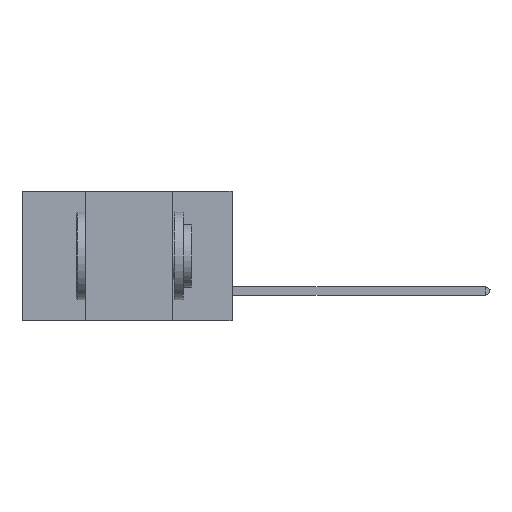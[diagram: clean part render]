
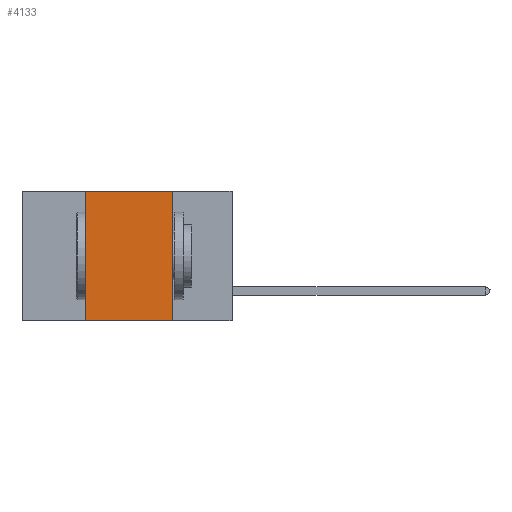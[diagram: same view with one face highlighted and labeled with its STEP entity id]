
A CAD part, left-side view. The second image highlights one B-rep face of the part: STEP entity #4133.
In plain terms, the highlighted planar face has unit normal (-1, 0, 0).
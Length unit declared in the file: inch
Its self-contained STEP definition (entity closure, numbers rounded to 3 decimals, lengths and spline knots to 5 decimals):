
#1001 = CARTESIAN_POINT ( 'NONE',  ( 0., 0.17, 0. ) ) ;
#1091 = ORIENTED_EDGE ( 'NONE', *, *, #10541, .T. ) ;
#1177 = EDGE_CURVE ( 'NONE', #11917, #10775, #2527, .T. ) ;
#1195 = CARTESIAN_POINT ( 'NONE',  ( 0., 0.6, 0. ) ) ;
#1341 = CARTESIAN_POINT ( 'NONE',  ( 0., 0.42, 0. ) ) ;
#2527 = LINE ( 'NONE', #1001, #4991 ) ;
#3161 = DIRECTION ( 'NONE',  ( 1., 0., 0. ) ) ;
#3175 = EDGE_LOOP ( 'NONE', ( #11600, #6607, #9332, #1091 ) ) ;
#3208 = VECTOR ( 'NONE', #3527, 39.37008 ) ;
#3527 = DIRECTION ( 'NONE',  ( 0., -1., 0. ) ) ;
#3568 = DIRECTION ( 'NONE',  ( 0., -1., 0. ) ) ;
#3571 = DIRECTION ( 'NONE',  ( 0., 0., 1. ) ) ;
#3637 = CARTESIAN_POINT ( 'NONE',  ( 0., 0.6, -0.37 ) ) ;
#3940 = DIRECTION ( 'NONE',  ( 0., 0., -1. ) ) ;
#4133 = ADVANCED_FACE ( 'NONE', ( #4643 ), #5069, .F. ) ;
#4355 = AXIS2_PLACEMENT_3D ( 'NONE', #1195, #3161, #6945 ) ;
#4589 = EDGE_CURVE ( 'NONE', #8487, #11917, #5397, .T. ) ;
#4643 = FACE_OUTER_BOUND ( 'NONE', #3175, .T. ) ;
#4991 = VECTOR ( 'NONE', #3940, 39.37008 ) ;
#5069 = PLANE ( 'NONE',  #4355 ) ;
#5106 = VECTOR ( 'NONE', #3568, 39.37008 ) ;
#5397 = LINE ( 'NONE', #11405, #3208 ) ;
#6426 = CARTESIAN_POINT ( 'NONE',  ( 0., 0.42, -0.37 ) ) ;
#6542 = VECTOR ( 'NONE', #3571, 39.37008 ) ;
#6607 = ORIENTED_EDGE ( 'NONE', *, *, #4589, .F. ) ;
#6945 = DIRECTION ( 'NONE',  ( 0., 0., -1. ) ) ;
#7598 = EDGE_CURVE ( 'NONE', #11365, #8487, #7765, .T. ) ;
#7765 = LINE ( 'NONE', #9453, #6542 ) ;
#8019 = CARTESIAN_POINT ( 'NONE',  ( 0., 0.17, -0.37 ) ) ;
#8487 = VERTEX_POINT ( 'NONE', #1341 ) ;
#9332 = ORIENTED_EDGE ( 'NONE', *, *, #7598, .F. ) ;
#9453 = CARTESIAN_POINT ( 'NONE',  ( 0., 0.42, 0. ) ) ;
#10318 = LINE ( 'NONE', #3637, #5106 ) ;
#10541 = EDGE_CURVE ( 'NONE', #11365, #10775, #10318, .T. ) ;
#10557 = CARTESIAN_POINT ( 'NONE',  ( 0., 0.17, 0. ) ) ;
#10775 = VERTEX_POINT ( 'NONE', #8019 ) ;
#11365 = VERTEX_POINT ( 'NONE', #6426 ) ;
#11405 = CARTESIAN_POINT ( 'NONE',  ( 0., 0.6, 0. ) ) ;
#11600 = ORIENTED_EDGE ( 'NONE', *, *, #1177, .F. ) ;
#11917 = VERTEX_POINT ( 'NONE', #10557 ) ;
